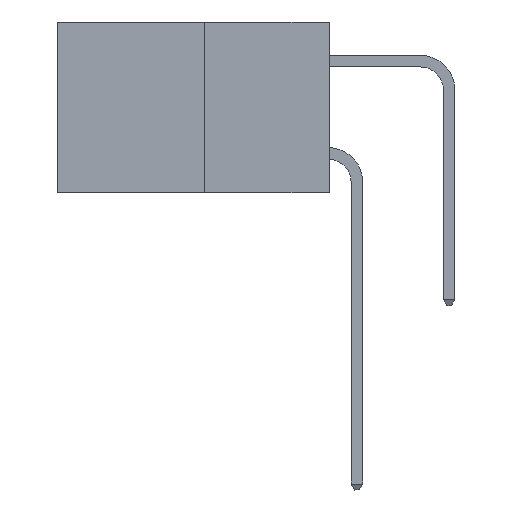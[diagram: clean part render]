
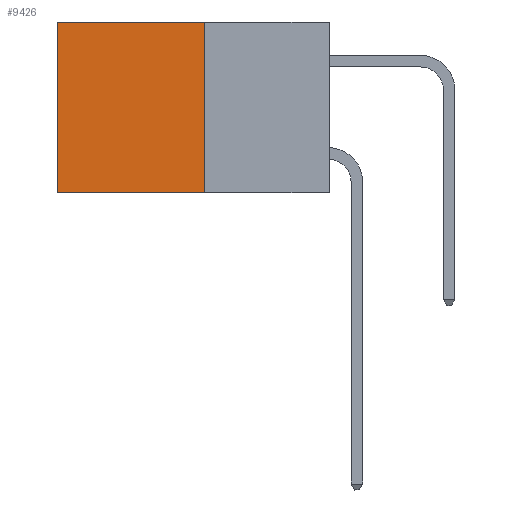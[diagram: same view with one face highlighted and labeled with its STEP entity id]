
A CAD part, left-side view. The second image highlights one B-rep face of the part: STEP entity #9426.
In plain terms, the highlighted planar face has unit normal (-1, 0, 0).
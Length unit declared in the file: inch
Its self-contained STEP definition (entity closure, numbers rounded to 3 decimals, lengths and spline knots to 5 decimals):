
#1910 = DIRECTION ( 'NONE',  ( 0., 0., -1. ) ) ;
#2453 = VECTOR ( 'NONE', #1910, 39.37008 ) ;
#2863 = EDGE_CURVE ( 'NONE', #21900, #19289, #8075, .T. ) ;
#3272 = VECTOR ( 'NONE', #18739, 39.37008 ) ;
#3489 = EDGE_CURVE ( 'NONE', #7990, #21900, #13898, .T. ) ;
#3602 = DIRECTION ( 'NONE',  ( 1., 0., 0. ) ) ;
#3976 = ORIENTED_EDGE ( 'NONE', *, *, #2863, .F. ) ;
#5294 = EDGE_LOOP ( 'NONE', ( #9677, #3976, #22618, #22377 ) ) ;
#7261 = CARTESIAN_POINT ( 'NONE',  ( 0.277, 0.27, -0.37 ) ) ;
#7725 = VERTEX_POINT ( 'NONE', #21015 ) ;
#7990 = VERTEX_POINT ( 'NONE', #12519 ) ;
#8075 = LINE ( 'NONE', #13927, #12483 ) ;
#9426 = ADVANCED_FACE ( 'NONE', ( #15088 ), #14812, .F. ) ;
#9677 = ORIENTED_EDGE ( 'NONE', *, *, #10182, .T. ) ;
#10182 = EDGE_CURVE ( 'NONE', #7725, #19289, #23446, .T. ) ;
#11744 = EDGE_CURVE ( 'NONE', #7990, #7725, #18149, .T. ) ;
#12483 = VECTOR ( 'NONE', #12774, 39.37008 ) ;
#12519 = CARTESIAN_POINT ( 'NONE',  ( 0.277, 0.27, 0. ) ) ;
#12668 = CARTESIAN_POINT ( 'NONE',  ( 0.277, 0.59, -0.37 ) ) ;
#12774 = DIRECTION ( 'NONE',  ( 0., 1., 0. ) ) ;
#13898 = LINE ( 'NONE', #16309, #23141 ) ;
#13927 = CARTESIAN_POINT ( 'NONE',  ( 0.277, 0.27, -0.37 ) ) ;
#14812 = PLANE ( 'NONE',  #21024 ) ;
#15088 = FACE_OUTER_BOUND ( 'NONE', #5294, .T. ) ;
#16104 = DIRECTION ( 'NONE',  ( 0., 0., -1. ) ) ;
#16309 = CARTESIAN_POINT ( 'NONE',  ( 0.277, 0.27, -0.37 ) ) ;
#16657 = DIRECTION ( 'NONE',  ( 0., 0., -1. ) ) ;
#16864 = CARTESIAN_POINT ( 'NONE',  ( 0.277, 0.27, 0. ) ) ;
#18149 = LINE ( 'NONE', #16864, #3272 ) ;
#18739 = DIRECTION ( 'NONE',  ( 0., 1., 0. ) ) ;
#19289 = VERTEX_POINT ( 'NONE', #12668 ) ;
#21015 = CARTESIAN_POINT ( 'NONE',  ( 0.277, 0.59, 0. ) ) ;
#21024 = AXIS2_PLACEMENT_3D ( 'NONE', #22178, #3602, #16657 ) ;
#21614 = CARTESIAN_POINT ( 'NONE',  ( 0.277, 0.59, -0.37 ) ) ;
#21900 = VERTEX_POINT ( 'NONE', #7261 ) ;
#22178 = CARTESIAN_POINT ( 'NONE',  ( 0.277, 0.27, -0.37 ) ) ;
#22377 = ORIENTED_EDGE ( 'NONE', *, *, #11744, .T. ) ;
#22618 = ORIENTED_EDGE ( 'NONE', *, *, #3489, .F. ) ;
#23141 = VECTOR ( 'NONE', #16104, 39.37008 ) ;
#23446 = LINE ( 'NONE', #21614, #2453 ) ;
